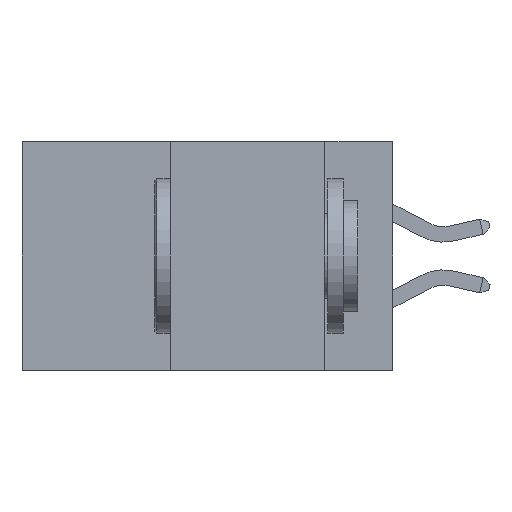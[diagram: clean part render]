
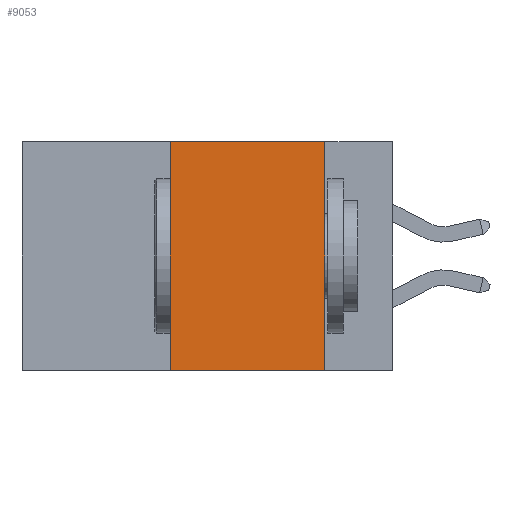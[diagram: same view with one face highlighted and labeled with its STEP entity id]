
A CAD part, left-side view. The second image highlights one B-rep face of the part: STEP entity #9053.
In plain terms, the highlighted planar face has unit normal (-1, 0, 0).
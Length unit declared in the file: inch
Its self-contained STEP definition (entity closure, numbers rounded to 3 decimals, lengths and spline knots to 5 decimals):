
#348 = CARTESIAN_POINT ( 'NONE',  ( 0., 0.6, 0. ) ) ;
#2470 = VERTEX_POINT ( 'NONE', #22065 ) ;
#2773 = EDGE_CURVE ( 'NONE', #11012, #2470, #32585, .T. ) ;
#2897 = DIRECTION ( 'NONE',  ( 0., 0., -1. ) ) ;
#3761 = LINE ( 'NONE', #21923, #29879 ) ;
#5385 = VECTOR ( 'NONE', #10647, 39.37008 ) ;
#8016 = VERTEX_POINT ( 'NONE', #18569 ) ;
#8361 = CARTESIAN_POINT ( 'NONE',  ( 0., 0.6, 0. ) ) ;
#8485 = CARTESIAN_POINT ( 'NONE',  ( 0., 0.36, -0.37 ) ) ;
#9053 = ADVANCED_FACE ( 'NONE', ( #17832 ), #15446, .F. ) ;
#9102 = AXIS2_PLACEMENT_3D ( 'NONE', #348, #17995, #2897 ) ;
#9127 = CARTESIAN_POINT ( 'NONE',  ( 0., 0.11, 0. ) ) ;
#9277 = DIRECTION ( 'NONE',  ( 0., 0., 1. ) ) ;
#10033 = VECTOR ( 'NONE', #18957, 39.37008 ) ;
#10647 = DIRECTION ( 'NONE',  ( 0., -1., 0. ) ) ;
#11012 = VERTEX_POINT ( 'NONE', #8485 ) ;
#12256 = VERTEX_POINT ( 'NONE', #20724 ) ;
#13082 = ORIENTED_EDGE ( 'NONE', *, *, #2773, .T. ) ;
#13337 = EDGE_CURVE ( 'NONE', #8016, #2470, #14797, .T. ) ;
#13847 = EDGE_LOOP ( 'NONE', ( #21458, #18590, #22238, #13082 ) ) ;
#14444 = LINE ( 'NONE', #8361, #5385 ) ;
#14797 = LINE ( 'NONE', #9127, #10033 ) ;
#15446 = PLANE ( 'NONE',  #9102 ) ;
#17832 = FACE_OUTER_BOUND ( 'NONE', #13847, .T. ) ;
#17995 = DIRECTION ( 'NONE',  ( 1., 0., 0. ) ) ;
#18290 = VECTOR ( 'NONE', #26334, 39.37008 ) ;
#18569 = CARTESIAN_POINT ( 'NONE',  ( 0., 0.11, 0. ) ) ;
#18590 = ORIENTED_EDGE ( 'NONE', *, *, #29081, .F. ) ;
#18957 = DIRECTION ( 'NONE',  ( 0., 0., -1. ) ) ;
#20724 = CARTESIAN_POINT ( 'NONE',  ( 0., 0.36, 0. ) ) ;
#21458 = ORIENTED_EDGE ( 'NONE', *, *, #13337, .F. ) ;
#21911 = EDGE_CURVE ( 'NONE', #11012, #12256, #3761, .T. ) ;
#21923 = CARTESIAN_POINT ( 'NONE',  ( 0., 0.36, 0. ) ) ;
#22065 = CARTESIAN_POINT ( 'NONE',  ( 0., 0.11, -0.37 ) ) ;
#22238 = ORIENTED_EDGE ( 'NONE', *, *, #21911, .F. ) ;
#26221 = CARTESIAN_POINT ( 'NONE',  ( 0., 0.6, -0.37 ) ) ;
#26334 = DIRECTION ( 'NONE',  ( 0., -1., 0. ) ) ;
#29081 = EDGE_CURVE ( 'NONE', #12256, #8016, #14444, .T. ) ;
#29879 = VECTOR ( 'NONE', #9277, 39.37008 ) ;
#32585 = LINE ( 'NONE', #26221, #18290 ) ;
